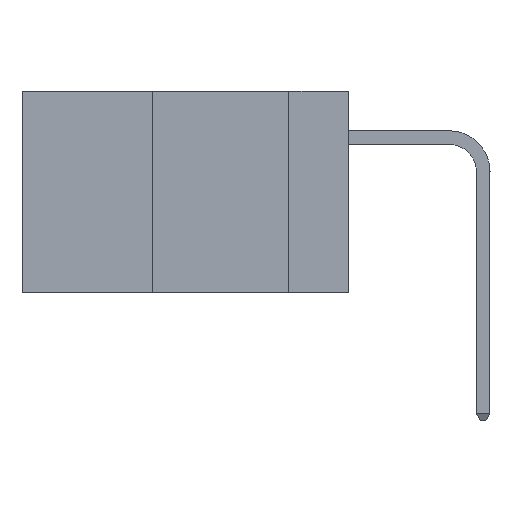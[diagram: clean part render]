
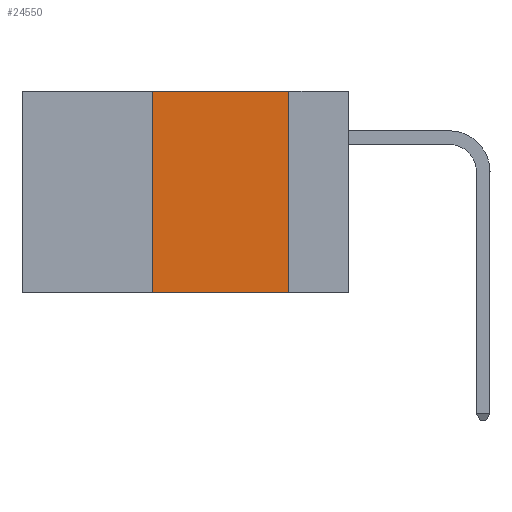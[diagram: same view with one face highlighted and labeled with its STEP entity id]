
A CAD part, left-side view. The second image highlights one B-rep face of the part: STEP entity #24550.
In plain terms, the highlighted planar face has unit normal (-1, 0, 0).
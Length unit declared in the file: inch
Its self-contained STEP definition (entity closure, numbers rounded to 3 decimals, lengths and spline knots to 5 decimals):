
#540 = VERTEX_POINT ( 'NONE', #17117 ) ;
#2730 = AXIS2_PLACEMENT_3D ( 'NONE', #25630, #36053, #8363 ) ;
#4671 = ORIENTED_EDGE ( 'NONE', *, *, #24163, .T. ) ;
#5380 = VECTOR ( 'NONE', #42117, 39.37008 ) ;
#5956 = VERTEX_POINT ( 'NONE', #34187 ) ;
#7152 = ORIENTED_EDGE ( 'NONE', *, *, #17107, .F. ) ;
#8363 = DIRECTION ( 'NONE',  ( 0., 0., -1. ) ) ;
#8578 = DIRECTION ( 'NONE',  ( 0., -1., 0. ) ) ;
#8870 = CARTESIAN_POINT ( 'NONE',  ( 0., 0.6, 0. ) ) ;
#9635 = LINE ( 'NONE', #10638, #5380 ) ;
#9885 = LINE ( 'NONE', #15690, #36428 ) ;
#10638 = CARTESIAN_POINT ( 'NONE',  ( 0., 0.6, -0.37 ) ) ;
#12110 = EDGE_CURVE ( 'NONE', #540, #42226, #9885, .T. ) ;
#12491 = ORIENTED_EDGE ( 'NONE', *, *, #12110, .F. ) ;
#12702 = VECTOR ( 'NONE', #36098, 39.37008 ) ;
#13376 = CARTESIAN_POINT ( 'NONE',  ( 0., 0.11, -0.37 ) ) ;
#14411 = VECTOR ( 'NONE', #8578, 39.37008 ) ;
#15690 = CARTESIAN_POINT ( 'NONE',  ( 0., 0.36, 0. ) ) ;
#17107 = EDGE_CURVE ( 'NONE', #5956, #19225, #43580, .T. ) ;
#17117 = CARTESIAN_POINT ( 'NONE',  ( 0., 0.36, -0.37 ) ) ;
#19225 = VERTEX_POINT ( 'NONE', #13376 ) ;
#19859 = FACE_OUTER_BOUND ( 'NONE', #26947, .T. ) ;
#23340 = EDGE_CURVE ( 'NONE', #42226, #5956, #34431, .T. ) ;
#24163 = EDGE_CURVE ( 'NONE', #540, #19225, #9635, .T. ) ;
#24550 = ADVANCED_FACE ( 'NONE', ( #19859 ), #29109, .F. ) ;
#25630 = CARTESIAN_POINT ( 'NONE',  ( 0., 0.6, 0. ) ) ;
#26947 = EDGE_LOOP ( 'NONE', ( #7152, #44222, #12491, #4671 ) ) ;
#28553 = CARTESIAN_POINT ( 'NONE',  ( 0., 0.11, 0. ) ) ;
#28902 = CARTESIAN_POINT ( 'NONE',  ( 0., 0.36, 0. ) ) ;
#29109 = PLANE ( 'NONE',  #2730 ) ;
#32632 = DIRECTION ( 'NONE',  ( 0., 0., 1. ) ) ;
#34187 = CARTESIAN_POINT ( 'NONE',  ( 0., 0.11, 0. ) ) ;
#34431 = LINE ( 'NONE', #8870, #14411 ) ;
#36053 = DIRECTION ( 'NONE',  ( 1., 0., 0. ) ) ;
#36098 = DIRECTION ( 'NONE',  ( 0., 0., -1. ) ) ;
#36428 = VECTOR ( 'NONE', #32632, 39.37008 ) ;
#42117 = DIRECTION ( 'NONE',  ( 0., -1., 0. ) ) ;
#42226 = VERTEX_POINT ( 'NONE', #28902 ) ;
#43580 = LINE ( 'NONE', #28553, #12702 ) ;
#44222 = ORIENTED_EDGE ( 'NONE', *, *, #23340, .F. ) ;
